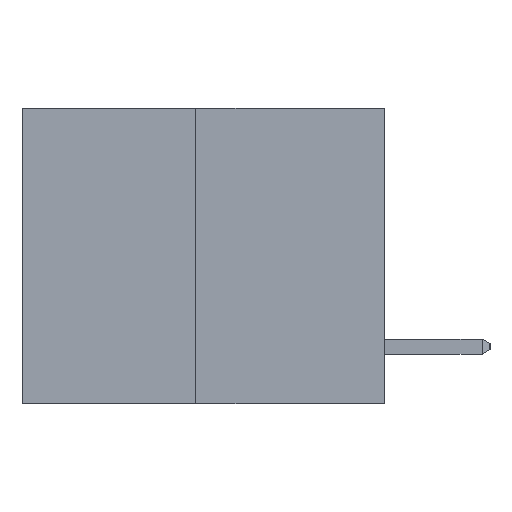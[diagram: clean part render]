
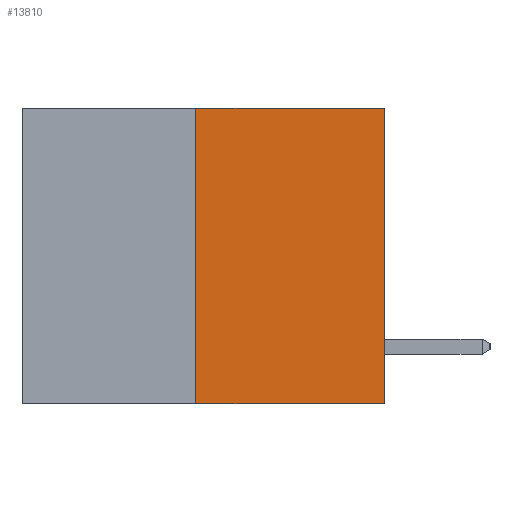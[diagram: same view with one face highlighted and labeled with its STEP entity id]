
A CAD part, left-side view. The second image highlights one B-rep face of the part: STEP entity #13810.
In plain terms, the highlighted planar face has unit normal (-1, 0, 0).
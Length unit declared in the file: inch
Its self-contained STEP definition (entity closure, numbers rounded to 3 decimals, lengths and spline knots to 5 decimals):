
#373 = CARTESIAN_POINT ( 'NONE',  ( 0., 0., 0. ) ) ;
#622 = VECTOR ( 'NONE', #4214, 39.37008 ) ;
#853 = LINE ( 'NONE', #373, #5565 ) ;
#945 = CARTESIAN_POINT ( 'NONE',  ( 0., 0.312, 0. ) ) ;
#1097 = DIRECTION ( 'NONE',  ( 1., 0., 0. ) ) ;
#1681 = EDGE_CURVE ( 'NONE', #10946, #12507, #4314, .T. ) ;
#2055 = EDGE_CURVE ( 'NONE', #10946, #8499, #7181, .T. ) ;
#2079 = ORIENTED_EDGE ( 'NONE', *, *, #2055, .T. ) ;
#2500 = FACE_OUTER_BOUND ( 'NONE', #8105, .T. ) ;
#3580 = VECTOR ( 'NONE', #11725, 39.37008 ) ;
#4166 = CARTESIAN_POINT ( 'NONE',  ( 0., 0.6, 0. ) ) ;
#4214 = DIRECTION ( 'NONE',  ( 0., -1., 0. ) ) ;
#4314 = LINE ( 'NONE', #12965, #12543 ) ;
#4426 = ORIENTED_EDGE ( 'NONE', *, *, #11466, .T. ) ;
#4714 = EDGE_CURVE ( 'NONE', #12507, #9415, #13798, .T. ) ;
#4915 = CARTESIAN_POINT ( 'NONE',  ( 0., 0.6, -0.49 ) ) ;
#5371 = CARTESIAN_POINT ( 'NONE',  ( 0., 0.6, 0. ) ) ;
#5565 = VECTOR ( 'NONE', #6668, 39.37008 ) ;
#6668 = DIRECTION ( 'NONE',  ( 0., 0., 1. ) ) ;
#7181 = LINE ( 'NONE', #4915, #622 ) ;
#7475 = ORIENTED_EDGE ( 'NONE', *, *, #4714, .F. ) ;
#7561 = ORIENTED_EDGE ( 'NONE', *, *, #1681, .F. ) ;
#7688 = PLANE ( 'NONE',  #11876 ) ;
#8105 = EDGE_LOOP ( 'NONE', ( #7561, #2079, #4426, #7475 ) ) ;
#8499 = VERTEX_POINT ( 'NONE', #11208 ) ;
#9069 = CARTESIAN_POINT ( 'NONE',  ( 0., 0.312, -0.49 ) ) ;
#9415 = VERTEX_POINT ( 'NONE', #10894 ) ;
#10820 = DIRECTION ( 'NONE',  ( 0., 0., -1. ) ) ;
#10894 = CARTESIAN_POINT ( 'NONE',  ( 0., 0., 0. ) ) ;
#10946 = VERTEX_POINT ( 'NONE', #9069 ) ;
#10969 = DIRECTION ( 'NONE',  ( 0., 0., 1. ) ) ;
#11208 = CARTESIAN_POINT ( 'NONE',  ( 0., 0., -0.49 ) ) ;
#11466 = EDGE_CURVE ( 'NONE', #8499, #9415, #853, .T. ) ;
#11725 = DIRECTION ( 'NONE',  ( 0., -1., 0. ) ) ;
#11876 = AXIS2_PLACEMENT_3D ( 'NONE', #5371, #1097, #10820 ) ;
#12507 = VERTEX_POINT ( 'NONE', #945 ) ;
#12543 = VECTOR ( 'NONE', #10969, 39.37008 ) ;
#12965 = CARTESIAN_POINT ( 'NONE',  ( 0., 0.312, -0.49 ) ) ;
#13798 = LINE ( 'NONE', #4166, #3580 ) ;
#13810 = ADVANCED_FACE ( 'NONE', ( #2500 ), #7688, .F. ) ;
